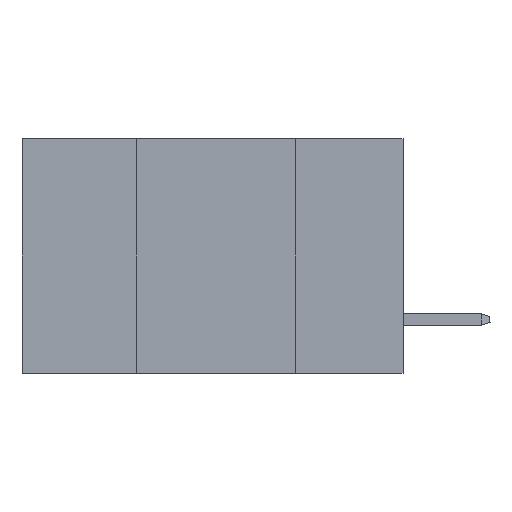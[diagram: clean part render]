
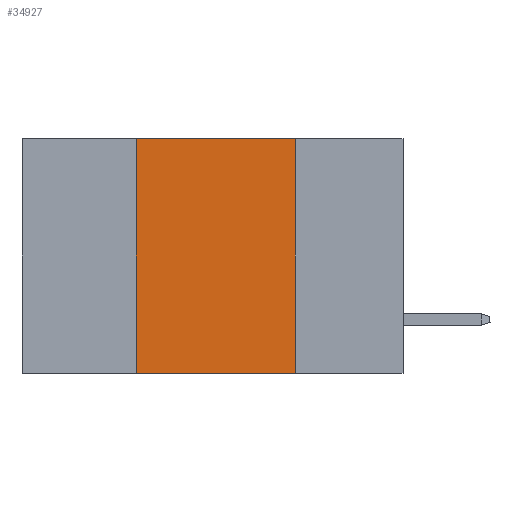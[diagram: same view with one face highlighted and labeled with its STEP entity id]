
A CAD part, left-side view. The second image highlights one B-rep face of the part: STEP entity #34927.
In plain terms, the highlighted planar face has unit normal (-1, 0, 0).
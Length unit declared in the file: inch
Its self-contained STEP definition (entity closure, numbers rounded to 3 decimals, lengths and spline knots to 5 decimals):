
#199 = EDGE_CURVE ( 'NONE', #3409, #20856, #37930, .T. ) ;
#3409 = VERTEX_POINT ( 'NONE', #39238 ) ;
#3415 = CARTESIAN_POINT ( 'NONE',  ( 0., 0.6, 0. ) ) ;
#6820 = ORIENTED_EDGE ( 'NONE', *, *, #199, .F. ) ;
#8757 = LINE ( 'NONE', #34986, #26273 ) ;
#10843 = CARTESIAN_POINT ( 'NONE',  ( 0., 0.17, 0. ) ) ;
#12130 = VECTOR ( 'NONE', #24105, 39.37008 ) ;
#14160 = PLANE ( 'NONE',  #30145 ) ;
#15078 = DIRECTION ( 'NONE',  ( 0., -1., 0. ) ) ;
#17043 = CARTESIAN_POINT ( 'NONE',  ( 0., 0.17, -0.37 ) ) ;
#17262 = CARTESIAN_POINT ( 'NONE',  ( 0., 0.6, 0. ) ) ;
#17839 = EDGE_CURVE ( 'NONE', #33624, #20856, #25436, .T. ) ;
#17912 = FACE_OUTER_BOUND ( 'NONE', #19833, .T. ) ;
#19692 = CARTESIAN_POINT ( 'NONE',  ( 0., 0.42, -0.37 ) ) ;
#19806 = VECTOR ( 'NONE', #26920, 39.37008 ) ;
#19833 = EDGE_LOOP ( 'NONE', ( #6820, #31370, #26073, #35331 ) ) ;
#20117 = EDGE_CURVE ( 'NONE', #33624, #30428, #8757, .T. ) ;
#20856 = VERTEX_POINT ( 'NONE', #17043 ) ;
#22188 = DIRECTION ( 'NONE',  ( 0., 0., 1. ) ) ;
#24105 = DIRECTION ( 'NONE',  ( 0., -1., 0. ) ) ;
#24309 = DIRECTION ( 'NONE',  ( 0., 0., -1. ) ) ;
#24329 = LINE ( 'NONE', #3415, #12130 ) ;
#24959 = DIRECTION ( 'NONE',  ( 1., 0., 0. ) ) ;
#25005 = CARTESIAN_POINT ( 'NONE',  ( 0., 0.6, -0.37 ) ) ;
#25436 = LINE ( 'NONE', #25005, #31465 ) ;
#26073 = ORIENTED_EDGE ( 'NONE', *, *, #20117, .F. ) ;
#26273 = VECTOR ( 'NONE', #22188, 39.37008 ) ;
#26920 = DIRECTION ( 'NONE',  ( 0., 0., -1. ) ) ;
#30145 = AXIS2_PLACEMENT_3D ( 'NONE', #17262, #24959, #24309 ) ;
#30428 = VERTEX_POINT ( 'NONE', #31055 ) ;
#31055 = CARTESIAN_POINT ( 'NONE',  ( 0., 0.42, 0. ) ) ;
#31370 = ORIENTED_EDGE ( 'NONE', *, *, #41229, .F. ) ;
#31465 = VECTOR ( 'NONE', #15078, 39.37008 ) ;
#33624 = VERTEX_POINT ( 'NONE', #19692 ) ;
#34927 = ADVANCED_FACE ( 'NONE', ( #17912 ), #14160, .F. ) ;
#34986 = CARTESIAN_POINT ( 'NONE',  ( 0., 0.42, 0. ) ) ;
#35331 = ORIENTED_EDGE ( 'NONE', *, *, #17839, .T. ) ;
#37930 = LINE ( 'NONE', #10843, #19806 ) ;
#39238 = CARTESIAN_POINT ( 'NONE',  ( 0., 0.17, 0. ) ) ;
#41229 = EDGE_CURVE ( 'NONE', #30428, #3409, #24329, .T. ) ;
